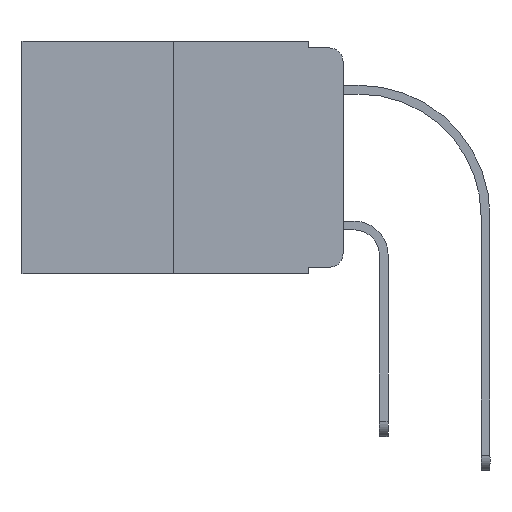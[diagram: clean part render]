
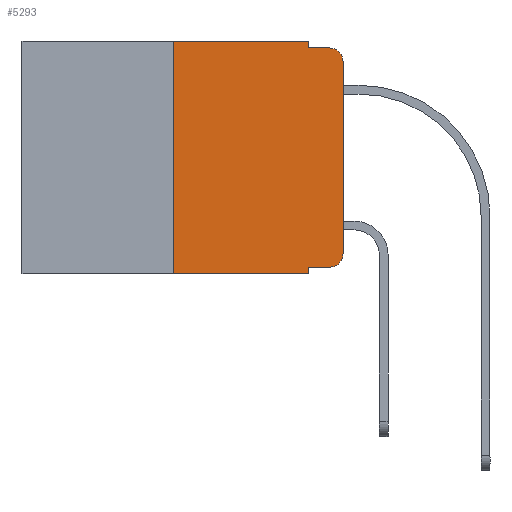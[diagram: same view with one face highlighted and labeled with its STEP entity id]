
A CAD part, left-side view. The second image highlights one B-rep face of the part: STEP entity #5293.
In plain terms, the highlighted planar face has unit normal (-1, 0, 0).
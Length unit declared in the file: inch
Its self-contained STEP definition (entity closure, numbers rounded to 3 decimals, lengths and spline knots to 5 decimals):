
#221 = LINE ( 'NONE', #7203, #3166 ) ;
#412 = CIRCLE ( 'NONE', #11175, 0.02 ) ;
#555 = CARTESIAN_POINT ( 'NONE',  ( 0., 0.051, -0.01 ) ) ;
#589 = VECTOR ( 'NONE', #8310, 39.37008 ) ;
#694 = DIRECTION ( 'NONE',  ( 0., -1., 0. ) ) ;
#831 = CARTESIAN_POINT ( 'NONE',  ( 0., 0.25, 0. ) ) ;
#849 = CARTESIAN_POINT ( 'NONE',  ( 0., 0.473, 0. ) ) ;
#996 = DIRECTION ( 'NONE',  ( -1., 0., 0. ) ) ;
#1039 = DIRECTION ( 'NONE',  ( 1., 0., 0. ) ) ;
#1058 = ORIENTED_EDGE ( 'NONE', *, *, #7277, .F. ) ;
#1308 = EDGE_CURVE ( 'NONE', #14309, #12516, #412, .T. ) ;
#1435 = DIRECTION ( 'NONE',  ( 0., -1., 0. ) ) ;
#1943 = LINE ( 'NONE', #849, #14027 ) ;
#2135 = CARTESIAN_POINT ( 'NONE',  ( 0., 0.473, 0. ) ) ;
#2249 = DIRECTION ( 'NONE',  ( 0., 0., -1. ) ) ;
#2352 = EDGE_CURVE ( 'NONE', #12467, #3744, #8226, .T. ) ;
#2529 = VECTOR ( 'NONE', #1435, 39.37008 ) ;
#2585 = DIRECTION ( 'NONE',  ( 0., 0., 1. ) ) ;
#2608 = ORIENTED_EDGE ( 'NONE', *, *, #6165, .F. ) ;
#2812 = VERTEX_POINT ( 'NONE', #15347 ) ;
#3036 = DIRECTION ( 'NONE',  ( 0., -1., 0. ) ) ;
#3166 = VECTOR ( 'NONE', #2585, 39.37008 ) ;
#3304 = CARTESIAN_POINT ( 'NONE',  ( 0., 0.02, -0.333 ) ) ;
#3454 = ORIENTED_EDGE ( 'NONE', *, *, #8962, .T. ) ;
#3473 = DIRECTION ( 'NONE',  ( 0., -1., 0. ) ) ;
#3744 = VERTEX_POINT ( 'NONE', #555 ) ;
#4383 = EDGE_CURVE ( 'NONE', #11193, #13010, #5233, .T. ) ;
#4524 = ORIENTED_EDGE ( 'NONE', *, *, #9600, .F. ) ;
#4581 = ORIENTED_EDGE ( 'NONE', *, *, #2352, .F. ) ;
#5233 = CIRCLE ( 'NONE', #9995, 0.02 ) ;
#5293 = ADVANCED_FACE ( 'NONE', ( #7932 ), #8162, .F. ) ;
#5376 = LINE ( 'NONE', #7884, #14771 ) ;
#5393 = EDGE_LOOP ( 'NONE', ( #12575, #10541, #4524, #4581, #12121, #2608, #11818, #1058, #3454, #7649 ) ) ;
#6165 = EDGE_CURVE ( 'NONE', #8331, #2812, #7008, .T. ) ;
#6296 = LINE ( 'NONE', #9823, #2529 ) ;
#6728 = LINE ( 'NONE', #7748, #12944 ) ;
#7008 = LINE ( 'NONE', #831, #15406 ) ;
#7203 = CARTESIAN_POINT ( 'NONE',  ( 0., 0., 0. ) ) ;
#7277 = EDGE_CURVE ( 'NONE', #14580, #12143, #6728, .T. ) ;
#7649 = ORIENTED_EDGE ( 'NONE', *, *, #1308, .T. ) ;
#7748 = CARTESIAN_POINT ( 'NONE',  ( 0., 0.051, 0. ) ) ;
#7884 = CARTESIAN_POINT ( 'NONE',  ( 0., 0.051, -0.333 ) ) ;
#7932 = FACE_OUTER_BOUND ( 'NONE', #5393, .T. ) ;
#7962 = CARTESIAN_POINT ( 'NONE',  ( 0., 0.051, -0.333 ) ) ;
#8162 = PLANE ( 'NONE',  #9026 ) ;
#8226 = LINE ( 'NONE', #10657, #589 ) ;
#8310 = DIRECTION ( 'NONE',  ( 0., 0., -1. ) ) ;
#8331 = VERTEX_POINT ( 'NONE', #9652 ) ;
#8361 = CARTESIAN_POINT ( 'NONE',  ( 0., 0.02, -0.01 ) ) ;
#8962 = EDGE_CURVE ( 'NONE', #14580, #14309, #5376, .T. ) ;
#9026 = AXIS2_PLACEMENT_3D ( 'NONE', #2135, #1039, #12950 ) ;
#9403 = CARTESIAN_POINT ( 'NONE',  ( 0., 0., -0.313 ) ) ;
#9600 = EDGE_CURVE ( 'NONE', #3744, #13010, #12732, .T. ) ;
#9652 = CARTESIAN_POINT ( 'NONE',  ( 0., 0.25, -0.343 ) ) ;
#9823 = CARTESIAN_POINT ( 'NONE',  ( 0., 0.473, -0.343 ) ) ;
#9995 = AXIS2_PLACEMENT_3D ( 'NONE', #11736, #996, #2249 ) ;
#10076 = CARTESIAN_POINT ( 'NONE',  ( 0., 0.02, -0.313 ) ) ;
#10541 = ORIENTED_EDGE ( 'NONE', *, *, #4383, .T. ) ;
#10657 = CARTESIAN_POINT ( 'NONE',  ( 0., 0.051, 0. ) ) ;
#11137 = CARTESIAN_POINT ( 'NONE',  ( 0., 0., -0.03 ) ) ;
#11175 = AXIS2_PLACEMENT_3D ( 'NONE', #10076, #11403, #12742 ) ;
#11193 = VERTEX_POINT ( 'NONE', #11137 ) ;
#11403 = DIRECTION ( 'NONE',  ( -1., 0., 0. ) ) ;
#11465 = EDGE_CURVE ( 'NONE', #2812, #12467, #1943, .T. ) ;
#11736 = CARTESIAN_POINT ( 'NONE',  ( 0., 0.02, -0.03 ) ) ;
#11818 = ORIENTED_EDGE ( 'NONE', *, *, #12144, .T. ) ;
#12121 = ORIENTED_EDGE ( 'NONE', *, *, #11465, .F. ) ;
#12143 = VERTEX_POINT ( 'NONE', #12169 ) ;
#12144 = EDGE_CURVE ( 'NONE', #8331, #12143, #6296, .T. ) ;
#12169 = CARTESIAN_POINT ( 'NONE',  ( 0., 0.051, -0.343 ) ) ;
#12455 = DIRECTION ( 'NONE',  ( 0., 0., -1. ) ) ;
#12467 = VERTEX_POINT ( 'NONE', #14480 ) ;
#12516 = VERTEX_POINT ( 'NONE', #9403 ) ;
#12575 = ORIENTED_EDGE ( 'NONE', *, *, #14357, .T. ) ;
#12732 = LINE ( 'NONE', #12881, #15291 ) ;
#12742 = DIRECTION ( 'NONE',  ( 0., 0., -1. ) ) ;
#12828 = DIRECTION ( 'NONE',  ( 0., 0., 1. ) ) ;
#12881 = CARTESIAN_POINT ( 'NONE',  ( 0., 0.051, -0.01 ) ) ;
#12944 = VECTOR ( 'NONE', #12455, 39.37008 ) ;
#12950 = DIRECTION ( 'NONE',  ( 0., 0., -1. ) ) ;
#13010 = VERTEX_POINT ( 'NONE', #8361 ) ;
#14027 = VECTOR ( 'NONE', #694, 39.37008 ) ;
#14309 = VERTEX_POINT ( 'NONE', #3304 ) ;
#14357 = EDGE_CURVE ( 'NONE', #12516, #11193, #221, .T. ) ;
#14480 = CARTESIAN_POINT ( 'NONE',  ( 0., 0.051, 0. ) ) ;
#14580 = VERTEX_POINT ( 'NONE', #7962 ) ;
#14771 = VECTOR ( 'NONE', #3036, 39.37008 ) ;
#15291 = VECTOR ( 'NONE', #3473, 39.37008 ) ;
#15347 = CARTESIAN_POINT ( 'NONE',  ( 0., 0.25, 0. ) ) ;
#15406 = VECTOR ( 'NONE', #12828, 39.37008 ) ;
